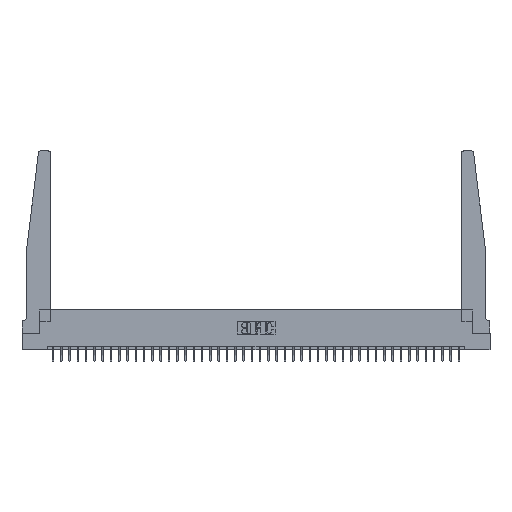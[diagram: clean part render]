
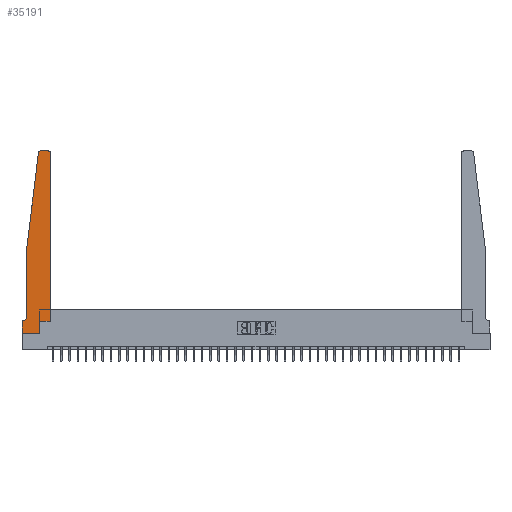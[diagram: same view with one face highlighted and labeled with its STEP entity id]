
A CAD part, top view. The second image highlights one B-rep face of the part: STEP entity #35191.
In plain terms, the highlighted planar face has unit normal (0, 0, 1).
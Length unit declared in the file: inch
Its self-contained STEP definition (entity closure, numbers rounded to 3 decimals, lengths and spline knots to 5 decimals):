
#1207 = DIRECTION ( 'NONE',  ( 0., 0., -1. ) ) ;
#1237 = CARTESIAN_POINT ( 'NONE',  ( 0.25, 2.75, 0.37 ) ) ;
#1904 = DIRECTION ( 'NONE',  ( 0., -1., 0. ) ) ;
#2015 = CARTESIAN_POINT ( 'NONE',  ( 0.065, 1.25, 0.37 ) ) ;
#3192 = CARTESIAN_POINT ( 'NONE',  ( 0.065, 1.25, 0.37 ) ) ;
#3559 = ORIENTED_EDGE ( 'NONE', *, *, #5580, .T. ) ;
#4430 = ORIENTED_EDGE ( 'NONE', *, *, #27285, .T. ) ;
#4553 = ORIENTED_EDGE ( 'NONE', *, *, #12709, .T. ) ;
#4878 = CARTESIAN_POINT ( 'NONE',  ( 0.015, 0.1875, 0.37 ) ) ;
#4910 = VERTEX_POINT ( 'NONE', #25495 ) ;
#5071 = AXIS2_PLACEMENT_3D ( 'NONE', #23879, #1207, #9625 ) ;
#5142 = VERTEX_POINT ( 'NONE', #3192 ) ;
#5203 = EDGE_CURVE ( 'NONE', #4910, #5142, #8264, .T. ) ;
#5552 = EDGE_CURVE ( 'NONE', #17073, #34151, #14423, .T. ) ;
#5580 = EDGE_CURVE ( 'NONE', #18009, #16305, #11789, .T. ) ;
#7533 = DIRECTION ( 'NONE',  ( 0., 1., 0. ) ) ;
#8238 = CARTESIAN_POINT ( 'NONE',  ( 0., 0., 0.37 ) ) ;
#8264 = LINE ( 'NONE', #2015, #23715 ) ;
#8439 = VERTEX_POINT ( 'NONE', #23729 ) ;
#8742 = ORIENTED_EDGE ( 'NONE', *, *, #5552, .T. ) ;
#8776 = VERTEX_POINT ( 'NONE', #14812 ) ;
#9118 = ORIENTED_EDGE ( 'NONE', *, *, #35232, .T. ) ;
#9365 = VECTOR ( 'NONE', #1904, 39.37008 ) ;
#9417 = DIRECTION ( 'NONE',  ( 1., 0., 0. ) ) ;
#9625 = DIRECTION ( 'NONE',  ( -1., 0., 0. ) ) ;
#9841 = CARTESIAN_POINT ( 'NONE',  ( 0.065, 1.25, 0.37 ) ) ;
#9929 = DIRECTION ( 'NONE',  ( 0., 0., 1. ) ) ;
#10513 = DIRECTION ( 'NONE',  ( 0., -1., 0. ) ) ;
#10597 = VECTOR ( 'NONE', #21665, 39.37008 ) ;
#11128 = LINE ( 'NONE', #1237, #28762 ) ;
#11671 = EDGE_CURVE ( 'NONE', #20367, #8776, #20370, .T. ) ;
#11698 = VECTOR ( 'NONE', #35774, 39.37008 ) ;
#11789 = LINE ( 'NONE', #16241, #17050 ) ;
#11915 = PLANE ( 'NONE',  #31340 ) ;
#12364 = LINE ( 'NONE', #16476, #10597 ) ;
#12408 = LINE ( 'NONE', #27115, #20734 ) ;
#12502 = CARTESIAN_POINT ( 'NONE',  ( 0.395, 2.72, 0.37 ) ) ;
#12709 = EDGE_CURVE ( 'NONE', #17624, #20367, #12408, .T. ) ;
#13969 = CARTESIAN_POINT ( 'NONE',  ( 0., 0.1875, 0.37 ) ) ;
#14423 = LINE ( 'NONE', #20436, #36105 ) ;
#14706 = DIRECTION ( 'NONE',  ( 0., 0., 1. ) ) ;
#14812 = CARTESIAN_POINT ( 'NONE',  ( 0.395, 2.75, 0.37 ) ) ;
#15175 = DIRECTION ( 'NONE',  ( 1., 0., 0. ) ) ;
#16241 = CARTESIAN_POINT ( 'NONE',  ( 0., 0., 0.37 ) ) ;
#16305 = VERTEX_POINT ( 'NONE', #8238 ) ;
#16404 = LINE ( 'NONE', #9841, #9365 ) ;
#16476 = CARTESIAN_POINT ( 'NONE',  ( 0., 0., 0.37 ) ) ;
#16712 = EDGE_CURVE ( 'NONE', #34151, #17624, #27989, .T. ) ;
#17050 = VECTOR ( 'NONE', #10513, 39.37008 ) ;
#17073 = VERTEX_POINT ( 'NONE', #29152 ) ;
#17250 = DIRECTION ( 'NONE',  ( -0.122, -0.992, 0. ) ) ;
#17410 = ORIENTED_EDGE ( 'NONE', *, *, #29270, .T. ) ;
#17435 = ORIENTED_EDGE ( 'NONE', *, *, #11671, .T. ) ;
#17624 = VERTEX_POINT ( 'NONE', #21020 ) ;
#18009 = VERTEX_POINT ( 'NONE', #13969 ) ;
#18613 = AXIS2_PLACEMENT_3D ( 'NONE', #12502, #32344, #9417 ) ;
#20367 = VERTEX_POINT ( 'NONE', #20649 ) ;
#20370 = CIRCLE ( 'NONE', #18613, 0.03 ) ;
#20436 = CARTESIAN_POINT ( 'NONE',  ( 0.2605, 0.18, 0.37 ) ) ;
#20649 = CARTESIAN_POINT ( 'NONE',  ( 0.425, 2.72, 0.37 ) ) ;
#20734 = VECTOR ( 'NONE', #7533, 39.37008 ) ;
#21020 = CARTESIAN_POINT ( 'NONE',  ( 0.425, 0.18, 0.37 ) ) ;
#21099 = ORIENTED_EDGE ( 'NONE', *, *, #16712, .T. ) ;
#21521 = CARTESIAN_POINT ( 'NONE',  ( 0.425, 0.18, 0.37 ) ) ;
#21562 = EDGE_LOOP ( 'NONE', ( #30104, #9118, #28104, #24695, #17410, #4430, #3559, #29995, #8742, #21099, #4553, #17435 ) ) ;
#21665 = DIRECTION ( 'NONE',  ( 1., 0., 0. ) ) ;
#21975 = EDGE_CURVE ( 'NONE', #8776, #8439, #11128, .T. ) ;
#23390 = CARTESIAN_POINT ( 'NONE',  ( 0.065, 0.1875, 0.37 ) ) ;
#23543 = DIRECTION ( 'NONE',  ( -1., 0., 0. ) ) ;
#23715 = VECTOR ( 'NONE', #17250, 39.37008 ) ;
#23729 = CARTESIAN_POINT ( 'NONE',  ( 0.27653, 2.75, 0.37 ) ) ;
#23879 = CARTESIAN_POINT ( 'NONE',  ( 0.015, 0.2375, 0.37 ) ) ;
#24296 = CARTESIAN_POINT ( 'NONE',  ( 0.065, 0.2375, 0.37 ) ) ;
#24695 = ORIENTED_EDGE ( 'NONE', *, *, #32343, .T. ) ;
#25295 = VERTEX_POINT ( 'NONE', #24296 ) ;
#25495 = CARTESIAN_POINT ( 'NONE',  ( 0.24675, 2.72367, 0.37 ) ) ;
#26049 = DIRECTION ( 'NONE',  ( 1., 0., 0. ) ) ;
#26745 = DIRECTION ( 'NONE',  ( 0., 1., 0. ) ) ;
#26780 = FACE_OUTER_BOUND ( 'NONE', #21562, .T. ) ;
#26835 = AXIS2_PLACEMENT_3D ( 'NONE', #32222, #9929, #15175 ) ;
#27115 = CARTESIAN_POINT ( 'NONE',  ( 0.425, 0.18, 0.37 ) ) ;
#27285 = EDGE_CURVE ( 'NONE', #34855, #18009, #35862, .T. ) ;
#27591 = CARTESIAN_POINT ( 'NONE',  ( 0.2605, 0.18, 0.37 ) ) ;
#27989 = LINE ( 'NONE', #21521, #11698 ) ;
#28104 = ORIENTED_EDGE ( 'NONE', *, *, #5203, .T. ) ;
#28319 = VECTOR ( 'NONE', #29319, 39.37008 ) ;
#28762 = VECTOR ( 'NONE', #23543, 39.37008 ) ;
#28897 = CARTESIAN_POINT ( 'NONE',  ( 0., 0.1875, 0.37 ) ) ;
#29152 = CARTESIAN_POINT ( 'NONE',  ( 0.2605, 0., 0.37 ) ) ;
#29270 = EDGE_CURVE ( 'NONE', #25295, #34855, #33495, .T. ) ;
#29319 = DIRECTION ( 'NONE',  ( -1., 0., 0. ) ) ;
#29995 = ORIENTED_EDGE ( 'NONE', *, *, #34156, .T. ) ;
#30104 = ORIENTED_EDGE ( 'NONE', *, *, #21975, .T. ) ;
#30351 = CIRCLE ( 'NONE', #26835, 0.03 ) ;
#31340 = AXIS2_PLACEMENT_3D ( 'NONE', #28897, #14706, #26049 ) ;
#32222 = CARTESIAN_POINT ( 'NONE',  ( 0.27653, 2.72, 0.37 ) ) ;
#32343 = EDGE_CURVE ( 'NONE', #5142, #25295, #16404, .T. ) ;
#32344 = DIRECTION ( 'NONE',  ( 0., 0., 1. ) ) ;
#33495 = CIRCLE ( 'NONE', #5071, 0.05 ) ;
#34151 = VERTEX_POINT ( 'NONE', #27591 ) ;
#34156 = EDGE_CURVE ( 'NONE', #16305, #17073, #12364, .T. ) ;
#34855 = VERTEX_POINT ( 'NONE', #4878 ) ;
#35191 = ADVANCED_FACE ( 'NONE', ( #26780 ), #11915, .T. ) ;
#35232 = EDGE_CURVE ( 'NONE', #8439, #4910, #30351, .T. ) ;
#35774 = DIRECTION ( 'NONE',  ( 1., 0., 0. ) ) ;
#35862 = LINE ( 'NONE', #23390, #28319 ) ;
#36105 = VECTOR ( 'NONE', #26745, 39.37008 ) ;
